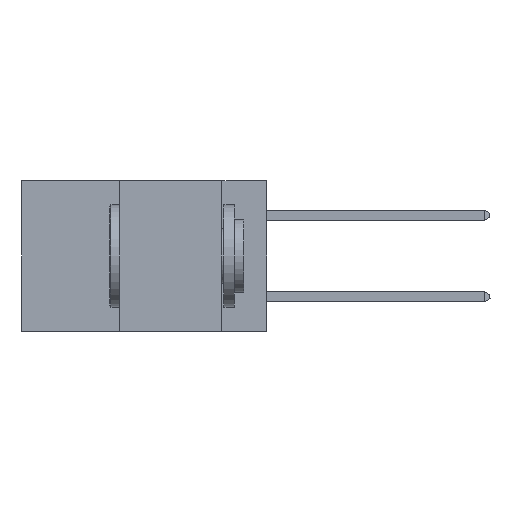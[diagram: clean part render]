
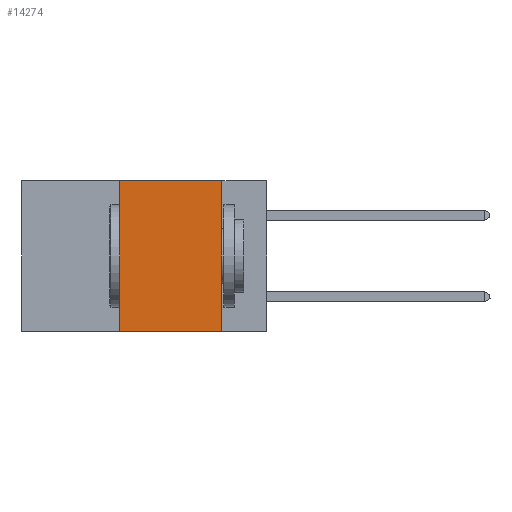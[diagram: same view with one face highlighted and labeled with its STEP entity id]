
A CAD part, left-side view. The second image highlights one B-rep face of the part: STEP entity #14274.
In plain terms, the highlighted planar face has unit normal (-1, 0, 0).
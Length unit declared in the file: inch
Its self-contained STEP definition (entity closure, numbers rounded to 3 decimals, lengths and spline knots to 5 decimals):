
#686 = VECTOR ( 'NONE', #2643, 39.37008 ) ;
#2497 = CARTESIAN_POINT ( 'NONE',  ( 0., 0.6, -0.37 ) ) ;
#2643 = DIRECTION ( 'NONE',  ( 0., -1., 0. ) ) ;
#2784 = LINE ( 'NONE', #32076, #686 ) ;
#3583 = DIRECTION ( 'NONE',  ( 0., 0., -1. ) ) ;
#3624 = DIRECTION ( 'NONE',  ( 0., 0., -1. ) ) ;
#3996 = EDGE_CURVE ( 'NONE', #6467, #21952, #2784, .T. ) ;
#5835 = DIRECTION ( 'NONE',  ( 0., -1., 0. ) ) ;
#6467 = VERTEX_POINT ( 'NONE', #32927 ) ;
#7399 = CARTESIAN_POINT ( 'NONE',  ( 0., 0.11, 0. ) ) ;
#10112 = CARTESIAN_POINT ( 'NONE',  ( 0., 0.6, 0. ) ) ;
#11908 = DIRECTION ( 'NONE',  ( 0., 0., 1. ) ) ;
#14160 = VECTOR ( 'NONE', #3624, 39.37008 ) ;
#14274 = ADVANCED_FACE ( 'NONE', ( #27746 ), #19950, .F. ) ;
#16976 = VERTEX_POINT ( 'NONE', #17150 ) ;
#17150 = CARTESIAN_POINT ( 'NONE',  ( 0., 0.11, -0.37 ) ) ;
#17837 = CARTESIAN_POINT ( 'NONE',  ( 0., 0.36, -0.37 ) ) ;
#19950 = PLANE ( 'NONE',  #36409 ) ;
#21952 = VERTEX_POINT ( 'NONE', #7399 ) ;
#22667 = VECTOR ( 'NONE', #11908, 39.37008 ) ;
#23373 = DIRECTION ( 'NONE',  ( 1., 0., 0. ) ) ;
#23414 = EDGE_CURVE ( 'NONE', #33207, #16976, #41924, .T. ) ;
#24433 = ORIENTED_EDGE ( 'NONE', *, *, #28812, .F. ) ;
#26384 = EDGE_CURVE ( 'NONE', #33207, #6467, #31289, .T. ) ;
#27746 = FACE_OUTER_BOUND ( 'NONE', #39877, .T. ) ;
#28512 = ORIENTED_EDGE ( 'NONE', *, *, #23414, .T. ) ;
#28812 = EDGE_CURVE ( 'NONE', #21952, #16976, #32582, .T. ) ;
#31289 = LINE ( 'NONE', #31531, #22667 ) ;
#31531 = CARTESIAN_POINT ( 'NONE',  ( 0., 0.36, 0. ) ) ;
#32076 = CARTESIAN_POINT ( 'NONE',  ( 0., 0.6, 0. ) ) ;
#32582 = LINE ( 'NONE', #33169, #14160 ) ;
#32927 = CARTESIAN_POINT ( 'NONE',  ( 0., 0.36, 0. ) ) ;
#33169 = CARTESIAN_POINT ( 'NONE',  ( 0., 0.11, 0. ) ) ;
#33207 = VERTEX_POINT ( 'NONE', #17837 ) ;
#33482 = VECTOR ( 'NONE', #5835, 39.37008 ) ;
#36043 = ORIENTED_EDGE ( 'NONE', *, *, #26384, .F. ) ;
#36409 = AXIS2_PLACEMENT_3D ( 'NONE', #10112, #23373, #3583 ) ;
#39877 = EDGE_LOOP ( 'NONE', ( #24433, #41488, #36043, #28512 ) ) ;
#41488 = ORIENTED_EDGE ( 'NONE', *, *, #3996, .F. ) ;
#41924 = LINE ( 'NONE', #2497, #33482 ) ;
